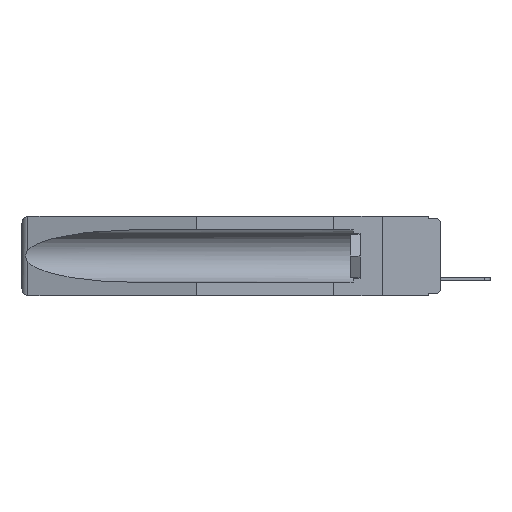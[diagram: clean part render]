
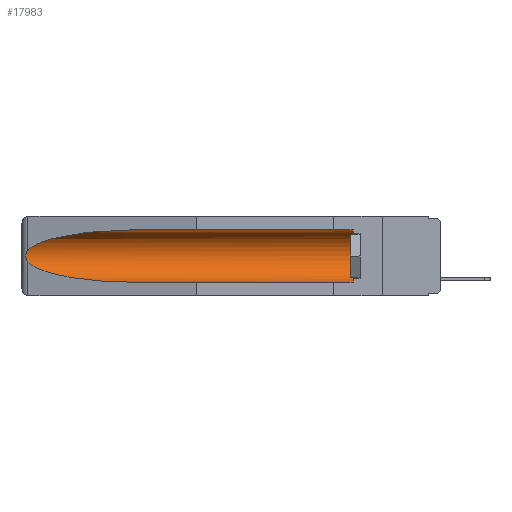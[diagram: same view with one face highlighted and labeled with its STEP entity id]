
A CAD part, left-side view. The second image highlights one B-rep face of the part: STEP entity #17983.
In plain terms, the highlighted cylindrical face has radius 2.857 mm (diameter 5.715 mm), a partial arc.
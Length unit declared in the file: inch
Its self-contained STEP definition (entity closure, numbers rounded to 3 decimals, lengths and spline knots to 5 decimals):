
#784 = ORIENTED_EDGE ( 'NONE', *, *, #26636, .T. ) ;
#970 = DIRECTION ( 'NONE',  ( 0., 0., 1. ) ) ;
#1250 = ORIENTED_EDGE ( 'NONE', *, *, #14551, .T. ) ;
#1727 = CARTESIAN_POINT ( 'NONE',  ( 0.2673, 1.5327, -0.16383 ) ) ;
#2151 = DIRECTION ( 'NONE',  ( 0., 0., 1. ) ) ;
#2293 = CARTESIAN_POINT ( 'NONE',  ( 0.155, 1.07973, -0.284 ) ) ;
#3138 = CARTESIAN_POINT ( 'NONE',  ( 0.26537, 1.52718, -0.14972 ) ) ;
#3409 = ORIENTED_EDGE ( 'NONE', *, *, #11828, .T. ) ;
#4001 = B_SPLINE_CURVE_WITH_KNOTS ( 'NONE', 3,
 ( #14376, #7772, #27105, #1727, #9847, #24652, #9941, #14296, #12052, #14206 ),
 .UNSPECIFIED., .F., .F.,
 ( 4, 2, 2, 2, 4 ),
 ( 0., 0.00029, 0.00058, 0.00087, 0.00117 ),
 .UNSPECIFIED. ) ;
#4211 = LINE ( 'NONE', #17202, #14208 ) ;
#5832 = CARTESIAN_POINT ( 'NONE',  ( 0.26537, 1.52718, -0.14972 ) ) ;
#7004 = AXIS2_PLACEMENT_3D ( 'NONE', #16731, #8300, #2151 ) ;
#7297 = VERTEX_POINT ( 'NONE', #21165 ) ;
#7443 = DIRECTION ( 'NONE',  ( 0., 1., 0. ) ) ;
#7515 = FACE_OUTER_BOUND ( 'NONE', #22981, .T. ) ;
#7772 = CARTESIAN_POINT ( 'NONE',  ( 0.26597, 1.52961, -0.15275 ) ) ;
#8119 = VERTEX_POINT ( 'NONE', #14990 ) ;
#8300 = DIRECTION ( 'NONE',  ( 0., 1., 0. ) ) ;
#8314 = EDGE_CURVE ( 'NONE', #13794, #7297, #4211, .T. ) ;
#8984 =( BOUNDED_CURVE ( )  B_SPLINE_CURVE ( 3, ( #13953, #9784, #16346, #5832 ),
 .UNSPECIFIED., .F., .F. ) 
 B_SPLINE_CURVE_WITH_KNOTS ( ( 4, 4 ),
 ( 4.71239, 6.08839 ),
 .UNSPECIFIED. ) 
 CURVE ( )  GEOMETRIC_REPRESENTATION_ITEM ( )  RATIONAL_B_SPLINE_CURVE ( ( 1., 0.848, 0.848, 1. ) ) 
 REPRESENTATION_ITEM ( '' )  );
#9441 = CARTESIAN_POINT ( 'NONE',  ( 0.155, 0.126, -0.1715 ) ) ;
#9660 = AXIS2_PLACEMENT_3D ( 'NONE', #9441, #24243, #970 ) ;
#9784 = CARTESIAN_POINT ( 'NONE',  ( 0.21114, 1.30732, -0.059 ) ) ;
#9847 = CARTESIAN_POINT ( 'NONE',  ( 0.2675, 1.53308, -0.16763 ) ) ;
#9941 = CARTESIAN_POINT ( 'NONE',  ( 0.2673, 1.53269, -0.17917 ) ) ;
#11325 = CARTESIAN_POINT ( 'NONE',  ( 0.26537, 1.52718, -0.19328 ) ) ;
#11682 = CARTESIAN_POINT ( 'NONE',  ( 0.155, 1.07973, -0.284 ) ) ;
#11828 = EDGE_CURVE ( 'NONE', #7297, #14430, #8984, .T. ) ;
#12052 = CARTESIAN_POINT ( 'NONE',  ( 0.26597, 1.5296, -0.19026 ) ) ;
#12385 = VERTEX_POINT ( 'NONE', #11325 ) ;
#13794 = VERTEX_POINT ( 'NONE', #22636 ) ;
#13953 = CARTESIAN_POINT ( 'NONE',  ( 0.155, 1.07973, -0.059 ) ) ;
#14206 = CARTESIAN_POINT ( 'NONE',  ( 0.26537, 1.52718, -0.19328 ) ) ;
#14208 = VECTOR ( 'NONE', #23664, 39.37008 ) ;
#14296 = CARTESIAN_POINT ( 'NONE',  ( 0.26655, 1.53094, -0.18657 ) ) ;
#14376 = CARTESIAN_POINT ( 'NONE',  ( 0.26537, 1.52718, -0.14972 ) ) ;
#14430 = VERTEX_POINT ( 'NONE', #3138 ) ;
#14551 = EDGE_CURVE ( 'NONE', #14430, #12385, #4001, .T. ) ;
#14602 = ORIENTED_EDGE ( 'NONE', *, *, #8314, .T. ) ;
#14990 = CARTESIAN_POINT ( 'NONE',  ( 0.155, 0.126, -0.284 ) ) ;
#15427 = ORIENTED_EDGE ( 'NONE', *, *, #17211, .T. ) ;
#16346 = CARTESIAN_POINT ( 'NONE',  ( 0.25451, 1.48313, -0.09465 ) ) ;
#16731 = CARTESIAN_POINT ( 'NONE',  ( 0.155, -0.30754, -0.1715 ) ) ;
#17202 = CARTESIAN_POINT ( 'NONE',  ( 0.155, -0.30754, -0.059 ) ) ;
#17211 = EDGE_CURVE ( 'NONE', #8119, #13794, #19854, .T. ) ;
#17983 = ADVANCED_FACE ( 'NONE', ( #7515 ), #22754, .F. ) ;
#18423 = EDGE_CURVE ( 'NONE', #8119, #26460, #25068, .T. ) ;
#19854 = CIRCLE ( 'NONE', #9660, 0.1125 ) ;
#20102 = CARTESIAN_POINT ( 'NONE',  ( 0.21114, 1.30732, -0.284 ) ) ;
#20278 = CARTESIAN_POINT ( 'NONE',  ( 0.26537, 1.52718, -0.19328 ) ) ;
#20286 =( BOUNDED_CURVE ( )  B_SPLINE_CURVE ( 3, ( #20278, #22142, #20102, #11682 ),
 .UNSPECIFIED., .F., .F. ) 
 B_SPLINE_CURVE_WITH_KNOTS ( ( 4, 4 ),
 ( 0.1948, 1.5708 ),
 .UNSPECIFIED. ) 
 CURVE ( )  GEOMETRIC_REPRESENTATION_ITEM ( )  RATIONAL_B_SPLINE_CURVE ( ( 1., 0.848, 0.848, 1. ) ) 
 REPRESENTATION_ITEM ( '' )  );
#20332 = CARTESIAN_POINT ( 'NONE',  ( 0.155, -0.30754, -0.284 ) ) ;
#21165 = CARTESIAN_POINT ( 'NONE',  ( 0.155, 1.07973, -0.059 ) ) ;
#22142 = CARTESIAN_POINT ( 'NONE',  ( 0.25451, 1.48313, -0.24835 ) ) ;
#22636 = CARTESIAN_POINT ( 'NONE',  ( 0.155, 0.126, -0.059 ) ) ;
#22754 = CYLINDRICAL_SURFACE ( 'NONE', #7004, 0.1125 ) ;
#22981 = EDGE_LOOP ( 'NONE', ( #3409, #1250, #784, #25444, #15427, #14602 ) ) ;
#23664 = DIRECTION ( 'NONE',  ( 0., 1., 0. ) ) ;
#24243 = DIRECTION ( 'NONE',  ( 0., -1., 0. ) ) ;
#24652 = CARTESIAN_POINT ( 'NONE',  ( 0.2675, 1.53308, -0.17534 ) ) ;
#25068 = LINE ( 'NONE', #20332, #27348 ) ;
#25444 = ORIENTED_EDGE ( 'NONE', *, *, #18423, .F. ) ;
#26460 = VERTEX_POINT ( 'NONE', #2293 ) ;
#26636 = EDGE_CURVE ( 'NONE', #12385, #26460, #20286, .T. ) ;
#27105 = CARTESIAN_POINT ( 'NONE',  ( 0.26654, 1.53092, -0.15636 ) ) ;
#27348 = VECTOR ( 'NONE', #7443, 39.37008 ) ;
